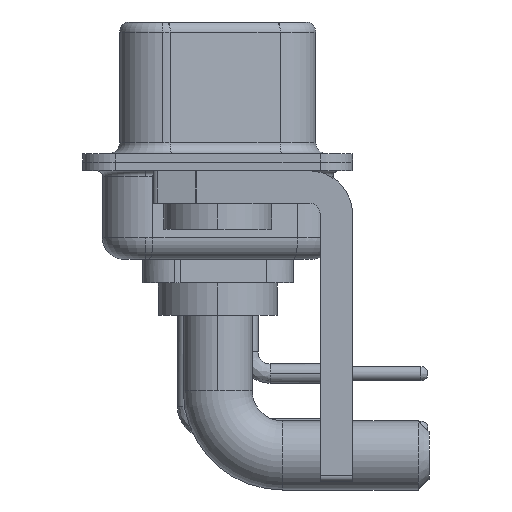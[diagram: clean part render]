
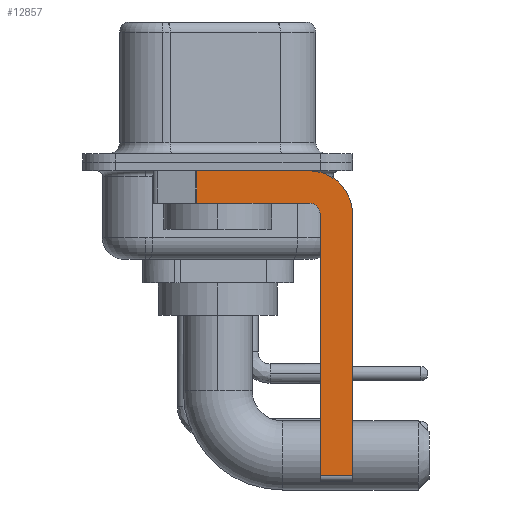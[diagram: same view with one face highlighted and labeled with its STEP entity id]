
A CAD part, left-side view. The second image highlights one B-rep face of the part: STEP entity #12857.
In plain terms, the highlighted planar face has unit normal (-1, 0, 0).
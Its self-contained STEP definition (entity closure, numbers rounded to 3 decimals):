
#977 = EDGE_CURVE ( 'NONE', #22808, #8260, #8086, .T. ) ;
#1225 = DIRECTION ( 'NONE',  ( 0., 0., 1. ) ) ;
#1251 = CARTESIAN_POINT ( 'NONE',  ( -2.9, -4.25, -0.4 ) ) ;
#1517 = VECTOR ( 'NONE', #1225, 1000. ) ;
#1904 = VECTOR ( 'NONE', #20536, 1000. ) ;
#2600 = DIRECTION ( 'NONE',  ( 0., 0., -1. ) ) ;
#2841 = VERTEX_POINT ( 'NONE', #1251 ) ;
#2926 = CIRCLE ( 'NONE', #10525, 2. ) ;
#3014 = DIRECTION ( 'NONE',  ( 1., 0., 0. ) ) ;
#3073 = VERTEX_POINT ( 'NONE', #8893 ) ;
#3207 = VERTEX_POINT ( 'NONE', #7068 ) ;
#3450 = DIRECTION ( 'NONE',  ( 0., -1., 0. ) ) ;
#4827 = CARTESIAN_POINT ( 'NONE',  ( -2.9, 0.978, -1.9 ) ) ;
#5232 = DIRECTION ( 'NONE',  ( 0., 0., -1. ) ) ;
#5245 = FACE_OUTER_BOUND ( 'NONE', #19831, .T. ) ;
#5458 = CARTESIAN_POINT ( 'NONE',  ( -2.9, -4.75, -2.4 ) ) ;
#5538 = DIRECTION ( 'NONE',  ( 0., -1., 0. ) ) ;
#5572 = LINE ( 'NONE', #10058, #25108 ) ;
#5957 = ORIENTED_EDGE ( 'NONE', *, *, #6721, .F. ) ;
#6639 = LINE ( 'NONE', #4827, #7886 ) ;
#6645 = CARTESIAN_POINT ( 'NONE',  ( -2.9, 0.978, -0.4 ) ) ;
#6721 = EDGE_CURVE ( 'NONE', #18908, #15304, #22984, .T. ) ;
#7068 = CARTESIAN_POINT ( 'NONE',  ( -2.9, -4.25, -1.9 ) ) ;
#7194 = CARTESIAN_POINT ( 'NONE',  ( -2.9, -4.25, -2.4 ) ) ;
#7297 = ORIENTED_EDGE ( 'NONE', *, *, #13130, .F. ) ;
#7886 = VECTOR ( 'NONE', #11009, 1000. ) ;
#7934 = CARTESIAN_POINT ( 'NONE',  ( -2.9, -6.25, -2.4 ) ) ;
#8086 = LINE ( 'NONE', #16410, #1517 ) ;
#8260 = VERTEX_POINT ( 'NONE', #5458 ) ;
#8429 = CARTESIAN_POINT ( 'NONE',  ( -2.9, -6.25, -14.55 ) ) ;
#8639 = ORIENTED_EDGE ( 'NONE', *, *, #977, .F. ) ;
#8893 = CARTESIAN_POINT ( 'NONE',  ( -2.9, 0.978, -1.9 ) ) ;
#9515 = VECTOR ( 'NONE', #19322, 1000. ) ;
#10058 = CARTESIAN_POINT ( 'NONE',  ( -2.9, -4.25, -14.55 ) ) ;
#10525 = AXIS2_PLACEMENT_3D ( 'NONE', #7194, #15932, #5232 ) ;
#10694 = EDGE_CURVE ( 'NONE', #3207, #3073, #20275, .T. ) ;
#10851 = VECTOR ( 'NONE', #5538, 1000. ) ;
#11009 = DIRECTION ( 'NONE',  ( 0., 0., -1. ) ) ;
#11500 = ORIENTED_EDGE ( 'NONE', *, *, #27542, .F. ) ;
#12132 = CARTESIAN_POINT ( 'NONE',  ( -2.9, 3., -0.4 ) ) ;
#12492 = CARTESIAN_POINT ( 'NONE',  ( -2.9, -4.25, -2.4 ) ) ;
#12610 = ORIENTED_EDGE ( 'NONE', *, *, #16856, .T. ) ;
#12857 = ADVANCED_FACE ( 'NONE', ( #5245 ), #13390, .F. ) ;
#13130 = EDGE_CURVE ( 'NONE', #8260, #3207, #19072, .T. ) ;
#13390 = PLANE ( 'NONE',  #23069 ) ;
#13644 = EDGE_CURVE ( 'NONE', #2841, #18908, #2926, .T. ) ;
#14576 = CARTESIAN_POINT ( 'NONE',  ( -2.9, -6.25, -2.4 ) ) ;
#14801 = EDGE_CURVE ( 'NONE', #23276, #3073, #6639, .T. ) ;
#14905 = DIRECTION ( 'NONE',  ( -1., 0., 0. ) ) ;
#15024 = AXIS2_PLACEMENT_3D ( 'NONE', #12492, #14905, #23464 ) ;
#15304 = VERTEX_POINT ( 'NONE', #8429 ) ;
#15932 = DIRECTION ( 'NONE',  ( 1., 0., 0. ) ) ;
#16410 = CARTESIAN_POINT ( 'NONE',  ( -2.9, -4.75, -14.8 ) ) ;
#16856 = EDGE_CURVE ( 'NONE', #22808, #15304, #5572, .T. ) ;
#17649 = CARTESIAN_POINT ( 'NONE',  ( -2.9, -4.25, -2.4 ) ) ;
#18887 = LINE ( 'NONE', #12132, #10851 ) ;
#18908 = VERTEX_POINT ( 'NONE', #14576 ) ;
#19072 = CIRCLE ( 'NONE', #15024, 0.5 ) ;
#19322 = DIRECTION ( 'NONE',  ( 0., 0., -1. ) ) ;
#19831 = EDGE_LOOP ( 'NONE', ( #11500, #25161, #23201, #7297, #8639, #12610, #5957, #21855 ) ) ;
#20275 = LINE ( 'NONE', #24588, #1904 ) ;
#20536 = DIRECTION ( 'NONE',  ( 0., 1., 0. ) ) ;
#21855 = ORIENTED_EDGE ( 'NONE', *, *, #13644, .F. ) ;
#22808 = VERTEX_POINT ( 'NONE', #25063 ) ;
#22984 = LINE ( 'NONE', #7934, #9515 ) ;
#23069 = AXIS2_PLACEMENT_3D ( 'NONE', #17649, #3014, #2600 ) ;
#23201 = ORIENTED_EDGE ( 'NONE', *, *, #10694, .F. ) ;
#23276 = VERTEX_POINT ( 'NONE', #6645 ) ;
#23464 = DIRECTION ( 'NONE',  ( 0., 0., 1. ) ) ;
#24588 = CARTESIAN_POINT ( 'NONE',  ( -2.9, -4.25, -1.9 ) ) ;
#25063 = CARTESIAN_POINT ( 'NONE',  ( -2.9, -4.75, -14.55 ) ) ;
#25108 = VECTOR ( 'NONE', #3450, 1000. ) ;
#25161 = ORIENTED_EDGE ( 'NONE', *, *, #14801, .T. ) ;
#27542 = EDGE_CURVE ( 'NONE', #23276, #2841, #18887, .T. ) ;
